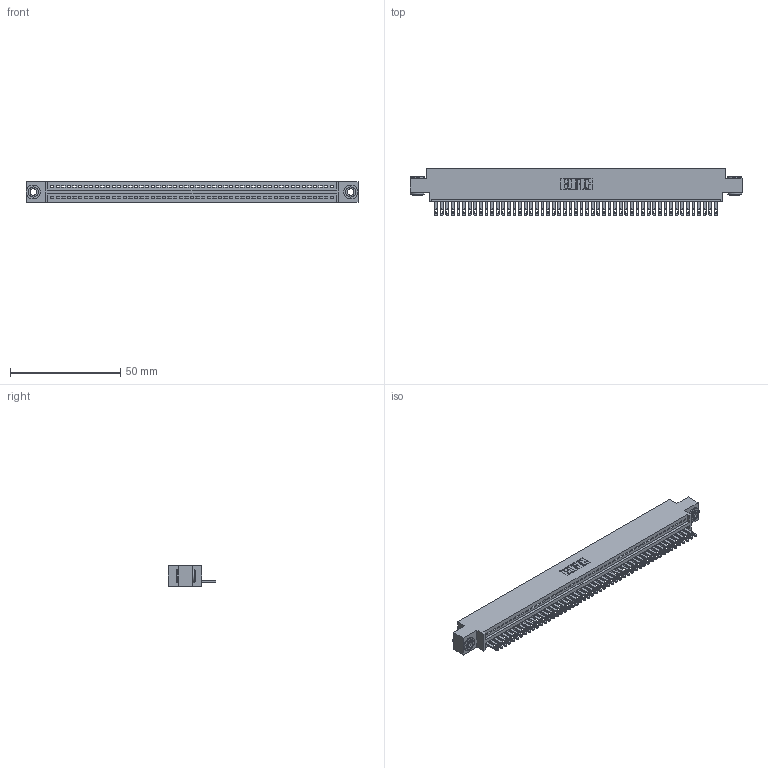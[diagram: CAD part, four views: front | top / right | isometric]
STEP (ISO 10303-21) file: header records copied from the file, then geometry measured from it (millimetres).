
FILE_DESCRIPTION (( 'STEP AP203' ), '1' );
FILE_NAME ('345-051-500-603.STEP', '2019-10-09T14:04:51', ( '' ), ( '' ), 'SwSTEP 2.0', 'SolidWorks 2016', '' );
FILE_SCHEMA (( 'CONFIG_CONTROL_DESIGN' ));
Length unit declared in the file: inch
Products named in the file (4): 345-051-500-603; 345 Part_0.170 Offset - 0.156 Dia-TH; 345-292-001_345-293-100; 345-250-002_345-250-002-102
Assembly tree (54 placements, depth 2):
  345-051-500-603
    345 Part_0.170 Offset - 0.156 Dia-TH
    345-292-001_345-293-100  x51
    345-250-002_345-250-002-102  x2
Bounding box: 150.75 x 21.51 x 9.4 mm (x, y, z)
Volume: 14329.6 mm3; surface area: 19620.6 mm2
Topology: 54 solids, 54 shells, 2922 faces, 8997 edges, 5994 vertices
Faces by surface type: plane 1828, cylinder 1086, cone 8
Entity records: 37884 total; most frequent: CARTESIAN_POINT 6540, ORIENTED_EDGE 6518, DIRECTION 5731, EDGE_CURVE 3259, LINE 2895, VECTOR 2895, VERTEX_POINT 2170, AXIS2_PLACEMENT_3D 1418
